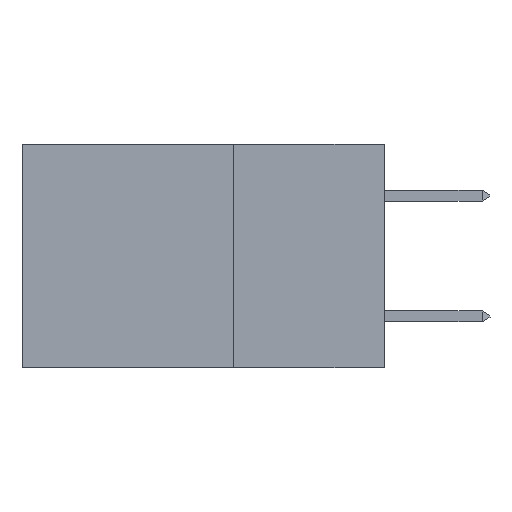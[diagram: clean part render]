
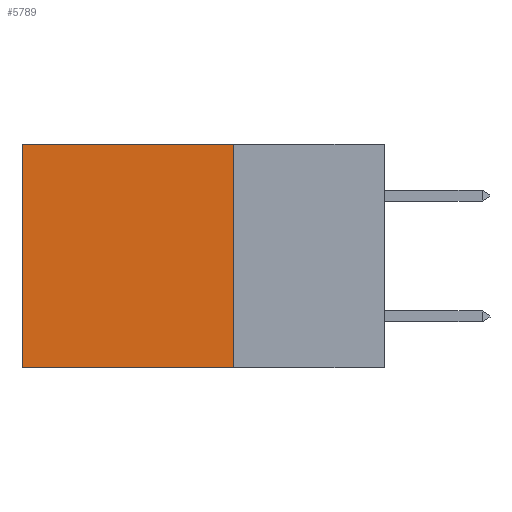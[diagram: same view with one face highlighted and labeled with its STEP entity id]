
A CAD part, left-side view. The second image highlights one B-rep face of the part: STEP entity #5789.
In plain terms, the highlighted planar face has unit normal (-1, 0, 0).
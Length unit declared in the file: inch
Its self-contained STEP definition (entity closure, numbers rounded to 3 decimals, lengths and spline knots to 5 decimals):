
#301 = VECTOR ( 'NONE', #3567, 39.37008 ) ;
#713 = EDGE_CURVE ( 'NONE', #16075, #2034, #10158, .T. ) ;
#981 = CARTESIAN_POINT ( 'NONE',  ( 0.2875, 0.25, -0.37 ) ) ;
#1752 = CARTESIAN_POINT ( 'NONE',  ( 0.2875, 0.25, 0. ) ) ;
#2034 = VERTEX_POINT ( 'NONE', #9072 ) ;
#2883 = LINE ( 'NONE', #10121, #6962 ) ;
#3567 = DIRECTION ( 'NONE',  ( 0., 1., 0. ) ) ;
#3849 = AXIS2_PLACEMENT_3D ( 'NONE', #4378, #16474, #6112 ) ;
#4378 = CARTESIAN_POINT ( 'NONE',  ( 0.2875, 0.25, 0. ) ) ;
#5789 = ADVANCED_FACE ( 'NONE', ( #13453 ), #14606, .F. ) ;
#6112 = DIRECTION ( 'NONE',  ( 0., 0., -1. ) ) ;
#6152 = CARTESIAN_POINT ( 'NONE',  ( 0.2875, 0.6, 0. ) ) ;
#6561 = ORIENTED_EDGE ( 'NONE', *, *, #6824, .F. ) ;
#6824 = EDGE_CURVE ( 'NONE', #20956, #21319, #2883, .T. ) ;
#6962 = VECTOR ( 'NONE', #11840, 39.37008 ) ;
#7633 = DIRECTION ( 'NONE',  ( 0., 0., -1. ) ) ;
#7882 = DIRECTION ( 'NONE',  ( 0., 0., -1. ) ) ;
#8198 = CARTESIAN_POINT ( 'NONE',  ( 0.2875, 0.6, -0.37 ) ) ;
#9072 = CARTESIAN_POINT ( 'NONE',  ( 0.2875, 0.6, 0. ) ) ;
#9886 = CARTESIAN_POINT ( 'NONE',  ( 0.2875, 0.25, 0. ) ) ;
#10121 = CARTESIAN_POINT ( 'NONE',  ( 0.2875, 0.25, -0.37 ) ) ;
#10158 = LINE ( 'NONE', #1752, #301 ) ;
#11840 = DIRECTION ( 'NONE',  ( 0., 1., 0. ) ) ;
#12384 = ORIENTED_EDGE ( 'NONE', *, *, #15172, .F. ) ;
#13453 = FACE_OUTER_BOUND ( 'NONE', #21243, .T. ) ;
#13832 = VECTOR ( 'NONE', #7882, 39.37008 ) ;
#14363 = LINE ( 'NONE', #6152, #13832 ) ;
#14606 = PLANE ( 'NONE',  #3849 ) ;
#14764 = ORIENTED_EDGE ( 'NONE', *, *, #18438, .T. ) ;
#15172 = EDGE_CURVE ( 'NONE', #16075, #20956, #19732, .T. ) ;
#16075 = VERTEX_POINT ( 'NONE', #9886 ) ;
#16178 = CARTESIAN_POINT ( 'NONE',  ( 0.2875, 0.25, 0. ) ) ;
#16474 = DIRECTION ( 'NONE',  ( 1., 0., 0. ) ) ;
#16822 = ORIENTED_EDGE ( 'NONE', *, *, #713, .T. ) ;
#18438 = EDGE_CURVE ( 'NONE', #2034, #21319, #14363, .T. ) ;
#19189 = VECTOR ( 'NONE', #7633, 39.37008 ) ;
#19732 = LINE ( 'NONE', #16178, #19189 ) ;
#20956 = VERTEX_POINT ( 'NONE', #981 ) ;
#21243 = EDGE_LOOP ( 'NONE', ( #14764, #6561, #12384, #16822 ) ) ;
#21319 = VERTEX_POINT ( 'NONE', #8198 ) ;
